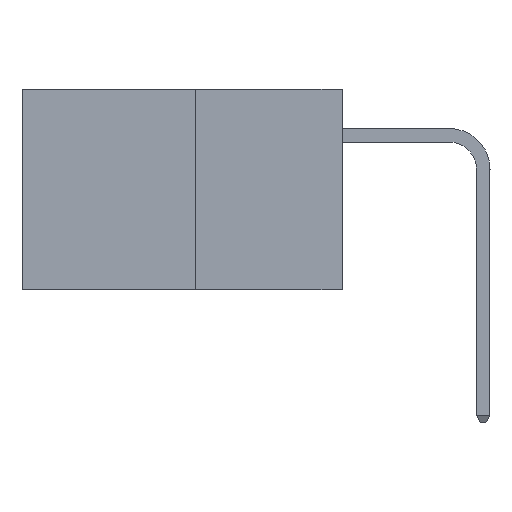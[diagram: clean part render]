
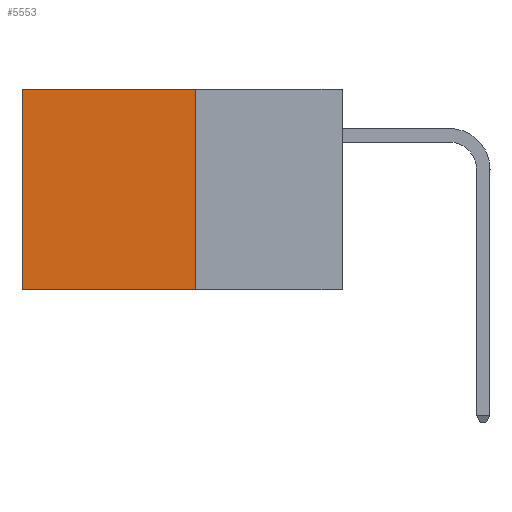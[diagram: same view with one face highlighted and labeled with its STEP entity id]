
A CAD part, left-side view. The second image highlights one B-rep face of the part: STEP entity #5553.
In plain terms, the highlighted planar face has unit normal (-1, 0, 0).
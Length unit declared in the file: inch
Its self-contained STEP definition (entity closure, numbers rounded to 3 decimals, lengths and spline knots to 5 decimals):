
#68 = DIRECTION ( 'NONE',  ( 0., 1., 0. ) ) ;
#276 = LINE ( 'NONE', #22973, #27851 ) ;
#376 = VERTEX_POINT ( 'NONE', #16011 ) ;
#2208 = VERTEX_POINT ( 'NONE', #10714 ) ;
#2557 = EDGE_CURVE ( 'NONE', #2208, #24950, #15498, .T. ) ;
#4000 = VECTOR ( 'NONE', #4954, 39.37008 ) ;
#4181 = EDGE_CURVE ( 'NONE', #24950, #25532, #22566, .T. ) ;
#4954 = DIRECTION ( 'NONE',  ( 0., 1., 0. ) ) ;
#5553 = ADVANCED_FACE ( 'NONE', ( #12228 ), #16985, .F. ) ;
#10375 = CARTESIAN_POINT ( 'NONE',  ( 0.277, 0.27, 0. ) ) ;
#10714 = CARTESIAN_POINT ( 'NONE',  ( 0.277, 0.27, 0. ) ) ;
#12228 = FACE_OUTER_BOUND ( 'NONE', #25753, .T. ) ;
#14057 = ORIENTED_EDGE ( 'NONE', *, *, #2557, .T. ) ;
#14354 = ORIENTED_EDGE ( 'NONE', *, *, #19313, .F. ) ;
#14792 = CARTESIAN_POINT ( 'NONE',  ( 0.277, 0.59, -0.37 ) ) ;
#15498 = LINE ( 'NONE', #10375, #4000 ) ;
#15836 = ORIENTED_EDGE ( 'NONE', *, *, #4181, .T. ) ;
#16011 = CARTESIAN_POINT ( 'NONE',  ( 0.277, 0.27, -0.37 ) ) ;
#16786 = VECTOR ( 'NONE', #22848, 39.37008 ) ;
#16919 = DIRECTION ( 'NONE',  ( 0., 0., -1. ) ) ;
#16925 = DIRECTION ( 'NONE',  ( 1., 0., 0. ) ) ;
#16985 = PLANE ( 'NONE',  #22990 ) ;
#17215 = CARTESIAN_POINT ( 'NONE',  ( 0.277, 0.27, -0.37 ) ) ;
#19313 = EDGE_CURVE ( 'NONE', #2208, #376, #276, .T. ) ;
#20753 = DIRECTION ( 'NONE',  ( 0., 0., -1. ) ) ;
#22300 = LINE ( 'NONE', #26178, #27413 ) ;
#22566 = LINE ( 'NONE', #23309, #16786 ) ;
#22848 = DIRECTION ( 'NONE',  ( 0., 0., -1. ) ) ;
#22973 = CARTESIAN_POINT ( 'NONE',  ( 0.277, 0.27, -0.37 ) ) ;
#22990 = AXIS2_PLACEMENT_3D ( 'NONE', #17215, #16925, #16919 ) ;
#23309 = CARTESIAN_POINT ( 'NONE',  ( 0.277, 0.59, -0.37 ) ) ;
#23796 = CARTESIAN_POINT ( 'NONE',  ( 0.277, 0.59, 0. ) ) ;
#24056 = ORIENTED_EDGE ( 'NONE', *, *, #26840, .F. ) ;
#24950 = VERTEX_POINT ( 'NONE', #23796 ) ;
#25532 = VERTEX_POINT ( 'NONE', #14792 ) ;
#25753 = EDGE_LOOP ( 'NONE', ( #15836, #24056, #14354, #14057 ) ) ;
#26178 = CARTESIAN_POINT ( 'NONE',  ( 0.277, 0.27, -0.37 ) ) ;
#26840 = EDGE_CURVE ( 'NONE', #376, #25532, #22300, .T. ) ;
#27413 = VECTOR ( 'NONE', #68, 39.37008 ) ;
#27851 = VECTOR ( 'NONE', #20753, 39.37008 ) ;
